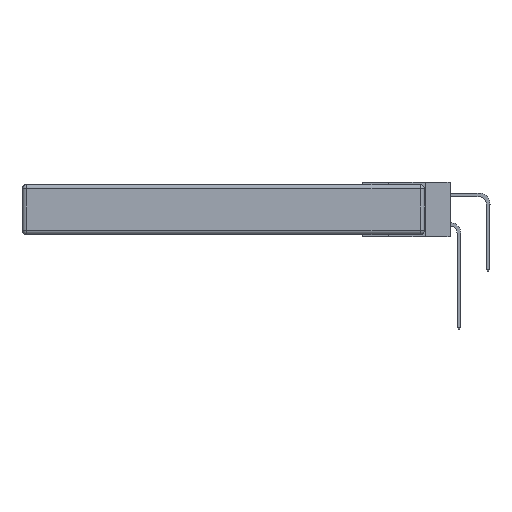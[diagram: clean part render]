
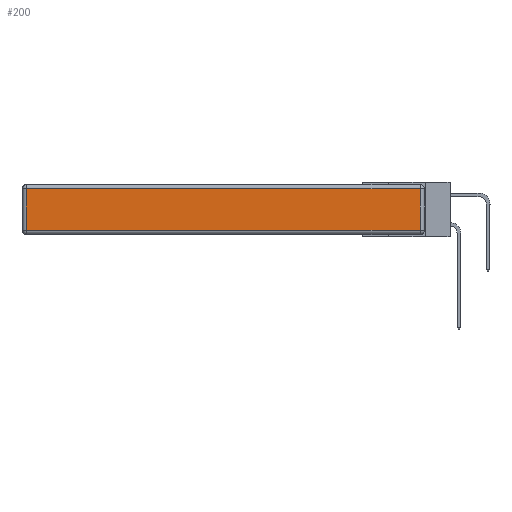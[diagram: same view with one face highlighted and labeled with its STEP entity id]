
A CAD part, left-side view. The second image highlights one B-rep face of the part: STEP entity #200.
In plain terms, the highlighted planar face has unit normal (-1, 0, 0).
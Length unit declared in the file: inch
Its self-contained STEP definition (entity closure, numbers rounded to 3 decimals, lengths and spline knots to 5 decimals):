
#200 = ADVANCED_FACE ( 'NONE', ( #20235 ), #10008, .T. ) ;
#4460 = VECTOR ( 'NONE', #29443, 39.37008 ) ;
#4586 = CARTESIAN_POINT ( 'NONE',  ( 0., 2.72, -0.343 ) ) ;
#4843 = DIRECTION ( 'NONE',  ( 0., -1., 0. ) ) ;
#6174 = EDGE_CURVE ( 'NONE', #10058, #14341, #23845, .T. ) ;
#6254 = VERTEX_POINT ( 'NONE', #16000 ) ;
#6476 = LINE ( 'NONE', #18957, #23602 ) ;
#7036 = EDGE_LOOP ( 'NONE', ( #20348, #29416, #25452, #7093 ) ) ;
#7093 = ORIENTED_EDGE ( 'NONE', *, *, #14728, .T. ) ;
#8751 = CARTESIAN_POINT ( 'NONE',  ( 0., 0.03, -0.313 ) ) ;
#9817 = CARTESIAN_POINT ( 'NONE',  ( 0., 0., -0.343 ) ) ;
#10008 = PLANE ( 'NONE',  #18222 ) ;
#10058 = VERTEX_POINT ( 'NONE', #8751 ) ;
#10111 = DIRECTION ( 'NONE',  ( -1., 0., 0. ) ) ;
#10412 = CARTESIAN_POINT ( 'NONE',  ( 0., 0.03, -0.343 ) ) ;
#13397 = LINE ( 'NONE', #4586, #18279 ) ;
#13535 = CARTESIAN_POINT ( 'NONE',  ( 0., 2.75, -0.03 ) ) ;
#13536 = VECTOR ( 'NONE', #25265, 39.37008 ) ;
#14341 = VERTEX_POINT ( 'NONE', #14448 ) ;
#14448 = CARTESIAN_POINT ( 'NONE',  ( 0., 0.03, -0.03 ) ) ;
#14728 = EDGE_CURVE ( 'NONE', #6254, #20570, #13397, .T. ) ;
#16000 = CARTESIAN_POINT ( 'NONE',  ( 0., 2.72, -0.03 ) ) ;
#18222 = AXIS2_PLACEMENT_3D ( 'NONE', #9817, #10111, #26772 ) ;
#18279 = VECTOR ( 'NONE', #18813, 39.37008 ) ;
#18813 = DIRECTION ( 'NONE',  ( 0., 0., -1. ) ) ;
#18957 = CARTESIAN_POINT ( 'NONE',  ( 0., 0., -0.313 ) ) ;
#20235 = FACE_OUTER_BOUND ( 'NONE', #7036, .T. ) ;
#20348 = ORIENTED_EDGE ( 'NONE', *, *, #29063, .T. ) ;
#20570 = VERTEX_POINT ( 'NONE', #28944 ) ;
#23602 = VECTOR ( 'NONE', #4843, 39.37008 ) ;
#23845 = LINE ( 'NONE', #10412, #4460 ) ;
#24309 = LINE ( 'NONE', #13535, #13536 ) ;
#25265 = DIRECTION ( 'NONE',  ( 0., 1., 0. ) ) ;
#25452 = ORIENTED_EDGE ( 'NONE', *, *, #29739, .T. ) ;
#26772 = DIRECTION ( 'NONE',  ( 0., 0., 1. ) ) ;
#28944 = CARTESIAN_POINT ( 'NONE',  ( 0., 2.72, -0.313 ) ) ;
#29063 = EDGE_CURVE ( 'NONE', #20570, #10058, #6476, .T. ) ;
#29416 = ORIENTED_EDGE ( 'NONE', *, *, #6174, .T. ) ;
#29443 = DIRECTION ( 'NONE',  ( 0., 0., 1. ) ) ;
#29739 = EDGE_CURVE ( 'NONE', #14341, #6254, #24309, .T. ) ;
